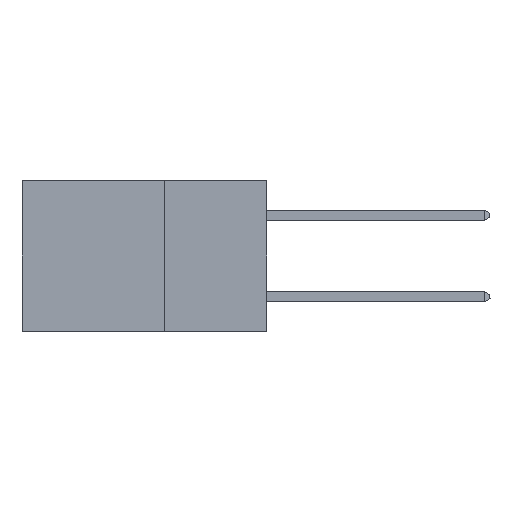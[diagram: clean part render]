
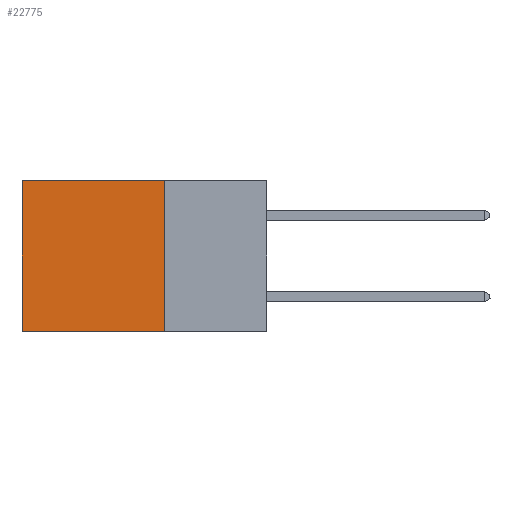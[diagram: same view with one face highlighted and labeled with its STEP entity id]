
A CAD part, left-side view. The second image highlights one B-rep face of the part: STEP entity #22775.
In plain terms, the highlighted planar face has unit normal (-1, 0, 0).
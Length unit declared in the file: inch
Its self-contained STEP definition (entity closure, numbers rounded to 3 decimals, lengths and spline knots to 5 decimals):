
#38 = ORIENTED_EDGE ( 'NONE', *, *, #865, .F. ) ;
#865 = EDGE_CURVE ( 'NONE', #8532, #24413, #5746, .T. ) ;
#1188 = VERTEX_POINT ( 'NONE', #7354 ) ;
#1250 = EDGE_CURVE ( 'NONE', #1188, #13467, #1308, .T. ) ;
#1308 = LINE ( 'NONE', #1836, #6408 ) ;
#1596 = DIRECTION ( 'NONE',  ( 0., 1., 0. ) ) ;
#1738 = CARTESIAN_POINT ( 'NONE',  ( 0.2875, 0.6, -0.37 ) ) ;
#1836 = CARTESIAN_POINT ( 'NONE',  ( 0.2875, 0.25, 0. ) ) ;
#2357 = CARTESIAN_POINT ( 'NONE',  ( 0.2875, 0.25, 0. ) ) ;
#2765 = DIRECTION ( 'NONE',  ( 0., 0., -1. ) ) ;
#3194 = VECTOR ( 'NONE', #19964, 39.37008 ) ;
#3972 = EDGE_CURVE ( 'NONE', #1188, #8532, #9645, .T. ) ;
#5114 = CARTESIAN_POINT ( 'NONE',  ( 0.2875, 0.6, 0. ) ) ;
#5746 = LINE ( 'NONE', #17445, #10189 ) ;
#6408 = VECTOR ( 'NONE', #1596, 39.37008 ) ;
#7354 = CARTESIAN_POINT ( 'NONE',  ( 0.2875, 0.25, 0. ) ) ;
#8532 = VERTEX_POINT ( 'NONE', #9387 ) ;
#8567 = EDGE_LOOP ( 'NONE', ( #15329, #38, #10471, #19256 ) ) ;
#9228 = PLANE ( 'NONE',  #25748 ) ;
#9387 = CARTESIAN_POINT ( 'NONE',  ( 0.2875, 0.25, -0.37 ) ) ;
#9645 = LINE ( 'NONE', #2357, #3194 ) ;
#10189 = VECTOR ( 'NONE', #18871, 39.37008 ) ;
#10471 = ORIENTED_EDGE ( 'NONE', *, *, #3972, .F. ) ;
#13467 = VERTEX_POINT ( 'NONE', #27037 ) ;
#13645 = CARTESIAN_POINT ( 'NONE',  ( 0.2875, 0.25, 0. ) ) ;
#14719 = FACE_OUTER_BOUND ( 'NONE', #8567, .T. ) ;
#15329 = ORIENTED_EDGE ( 'NONE', *, *, #18489, .T. ) ;
#15882 = DIRECTION ( 'NONE',  ( 1., 0., 0. ) ) ;
#16585 = VECTOR ( 'NONE', #24944, 39.37008 ) ;
#17445 = CARTESIAN_POINT ( 'NONE',  ( 0.2875, 0.25, -0.37 ) ) ;
#18489 = EDGE_CURVE ( 'NONE', #13467, #24413, #21797, .T. ) ;
#18871 = DIRECTION ( 'NONE',  ( 0., 1., 0. ) ) ;
#19256 = ORIENTED_EDGE ( 'NONE', *, *, #1250, .T. ) ;
#19964 = DIRECTION ( 'NONE',  ( 0., 0., -1. ) ) ;
#21797 = LINE ( 'NONE', #5114, #16585 ) ;
#22775 = ADVANCED_FACE ( 'NONE', ( #14719 ), #9228, .F. ) ;
#24413 = VERTEX_POINT ( 'NONE', #1738 ) ;
#24944 = DIRECTION ( 'NONE',  ( 0., 0., -1. ) ) ;
#25748 = AXIS2_PLACEMENT_3D ( 'NONE', #13645, #15882, #2765 ) ;
#27037 = CARTESIAN_POINT ( 'NONE',  ( 0.2875, 0.6, 0. ) ) ;
